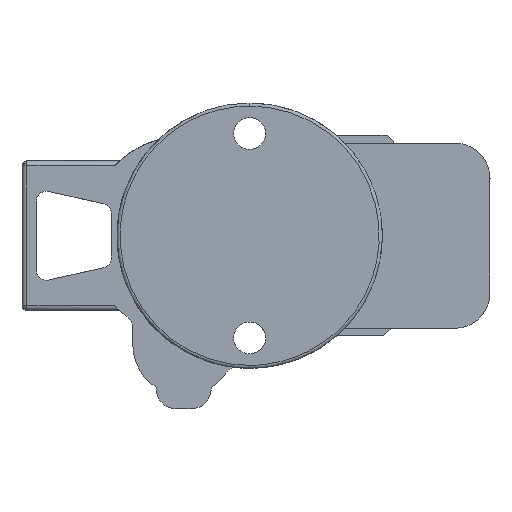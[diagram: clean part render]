
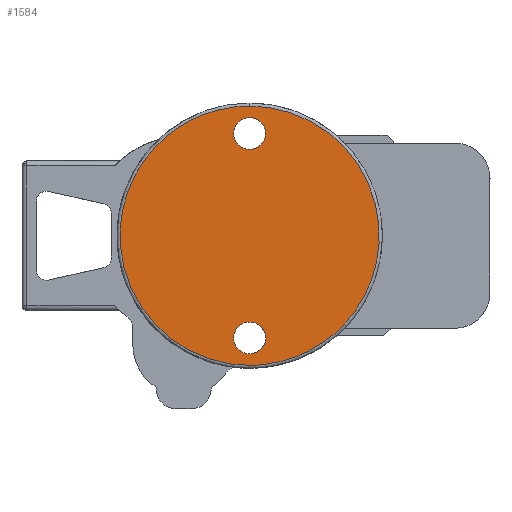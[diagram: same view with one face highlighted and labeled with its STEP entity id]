
A CAD part, left-side view. The second image highlights one B-rep face of the part: STEP entity #1584.
In plain terms, the highlighted planar face has unit normal (-1, 0, 0).
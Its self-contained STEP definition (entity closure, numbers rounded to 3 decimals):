
#74 = DIRECTION ( 'NONE',  ( 0., 0., -1. ) ) ;
#78 = VERTEX_POINT ( 'NONE', #683 ) ;
#122 = ORIENTED_EDGE ( 'NONE', *, *, #135, .F. ) ;
#135 = EDGE_CURVE ( 'NONE', #78, #2031, #2681, .T. ) ;
#228 = CARTESIAN_POINT ( 'NONE',  ( -218.682, 34.658, -22.7 ) ) ;
#279 = CARTESIAN_POINT ( 'NONE',  ( -218.682, 34.658, 18.3 ) ) ;
#391 = DIRECTION ( 'NONE',  ( -1., 0., 0. ) ) ;
#437 = CARTESIAN_POINT ( 'NONE',  ( -218.682, 34.658, -16.3 ) ) ;
#619 =( BOUNDED_CURVE ( )  B_SPLINE_CURVE ( 3, ( #1384, #3338, #1368, #3068 ),
 .UNSPECIFIED., .F., .T. ) 
 B_SPLINE_CURVE_WITH_KNOTS ( ( 4, 4 ),
 ( 0.876, 1.376 ),
 .UNSPECIFIED. ) 
 CURVE ( )  GEOMETRIC_REPRESENTATION_ITEM ( )  RATIONAL_B_SPLINE_CURVE ( ( 1., 0.333, 0.333, 1. ) ) 
 REPRESENTATION_ITEM ( '' )  );
#683 = CARTESIAN_POINT ( 'NONE',  ( -218.682, 34.658, 24.7 ) ) ;
#753 = AXIS2_PLACEMENT_3D ( 'NONE', #2430, #1034, #2156 ) ;
#888 = AXIS2_PLACEMENT_3D ( 'NONE', #3192, #2886, #1496 ) ;
#916 = DIRECTION ( 'NONE',  ( 0., 0., -1. ) ) ;
#926 = EDGE_CURVE ( 'NONE', #2140, #1071, #619, .T. ) ;
#1034 = DIRECTION ( 'NONE',  ( -1., 0., 0. ) ) ;
#1071 = VERTEX_POINT ( 'NONE', #3484 ) ;
#1086 = EDGE_LOOP ( 'NONE', ( #3415, #3290 ) ) ;
#1128 = CARTESIAN_POINT ( 'NONE',  ( -218.682, 34.658, 21.5 ) ) ;
#1136 = DIRECTION ( 'NONE',  ( 0., 0., -1. ) ) ;
#1143 = ORIENTED_EDGE ( 'NONE', *, *, #3253, .F. ) ;
#1180 = FACE_BOUND ( 'NONE', #1340, .T. ) ;
#1198 = PLANE ( 'NONE',  #3098 ) ;
#1291 = EDGE_CURVE ( 'NONE', #1765, #1603, #2693, .T. ) ;
#1315 =( BOUNDED_CURVE ( )  B_SPLINE_CURVE ( 3, ( #3286, #3069, #3339, #2214 ),
 .UNSPECIFIED., .F., .T. ) 
 B_SPLINE_CURVE_WITH_KNOTS ( ( 4, 4 ),
 ( 0.376, 0.876 ),
 .UNSPECIFIED. ) 
 CURVE ( )  GEOMETRIC_REPRESENTATION_ITEM ( )  RATIONAL_B_SPLINE_CURVE ( ( 1., 0.333, 0.333, 1. ) ) 
 REPRESENTATION_ITEM ( '' )  );
#1340 = EDGE_LOOP ( 'NONE', ( #122, #2192 ) ) ;
#1368 = CARTESIAN_POINT ( 'NONE',  ( -218.682, 86.64, 26.991 ) ) ;
#1384 = CARTESIAN_POINT ( 'NONE',  ( -218.682, 34.658, -24.991 ) ) ;
#1496 = DIRECTION ( 'NONE',  ( 0., 0., -1. ) ) ;
#1584 = ADVANCED_FACE ( 'NONE', ( #2590, #1180, #2296 ), #1198, .F. ) ;
#1603 = VERTEX_POINT ( 'NONE', #437 ) ;
#1614 = CARTESIAN_POINT ( 'NONE',  ( -218.682, 34.658, -24.991 ) ) ;
#1765 = VERTEX_POINT ( 'NONE', #228 ) ;
#1886 = CIRCLE ( 'NONE', #888, 3.2 ) ;
#2031 = VERTEX_POINT ( 'NONE', #279 ) ;
#2140 = VERTEX_POINT ( 'NONE', #1614 ) ;
#2156 = DIRECTION ( 'NONE',  ( 0., 0., -1. ) ) ;
#2160 = AXIS2_PLACEMENT_3D ( 'NONE', #3302, #3014, #1136 ) ;
#2182 = AXIS2_PLACEMENT_3D ( 'NONE', #1128, #391, #74 ) ;
#2192 = ORIENTED_EDGE ( 'NONE', *, *, #2774, .F. ) ;
#2214 = CARTESIAN_POINT ( 'NONE',  ( -218.682, 34.658, -24.991 ) ) ;
#2296 = FACE_BOUND ( 'NONE', #2443, .T. ) ;
#2311 = CARTESIAN_POINT ( 'NONE',  ( -218.682, 8.067, 1. ) ) ;
#2424 = ORIENTED_EDGE ( 'NONE', *, *, #1291, .F. ) ;
#2430 = CARTESIAN_POINT ( 'NONE',  ( -218.682, 34.658, -19.5 ) ) ;
#2443 = EDGE_LOOP ( 'NONE', ( #1143, #2424 ) ) ;
#2485 = EDGE_CURVE ( 'NONE', #1071, #2140, #1315, .T. ) ;
#2590 = FACE_OUTER_BOUND ( 'NONE', #1086, .T. ) ;
#2681 = CIRCLE ( 'NONE', #2160, 3.2 ) ;
#2693 = CIRCLE ( 'NONE', #753, 3.2 ) ;
#2774 = EDGE_CURVE ( 'NONE', #2031, #78, #3518, .T. ) ;
#2886 = DIRECTION ( 'NONE',  ( -1., 0., 0. ) ) ;
#3014 = DIRECTION ( 'NONE',  ( -1., 0., 0. ) ) ;
#3068 = CARTESIAN_POINT ( 'NONE',  ( -218.682, 34.658, 26.991 ) ) ;
#3069 = CARTESIAN_POINT ( 'NONE',  ( -218.682, -17.323, 26.991 ) ) ;
#3098 = AXIS2_PLACEMENT_3D ( 'NONE', #2311, #3422, #916 ) ;
#3192 = CARTESIAN_POINT ( 'NONE',  ( -218.682, 34.658, -19.5 ) ) ;
#3253 = EDGE_CURVE ( 'NONE', #1603, #1765, #1886, .T. ) ;
#3286 = CARTESIAN_POINT ( 'NONE',  ( -218.682, 34.658, 26.991 ) ) ;
#3290 = ORIENTED_EDGE ( 'NONE', *, *, #926, .F. ) ;
#3302 = CARTESIAN_POINT ( 'NONE',  ( -218.682, 34.658, 21.5 ) ) ;
#3338 = CARTESIAN_POINT ( 'NONE',  ( -218.682, 86.64, -24.991 ) ) ;
#3339 = CARTESIAN_POINT ( 'NONE',  ( -218.682, -17.323, -24.991 ) ) ;
#3415 = ORIENTED_EDGE ( 'NONE', *, *, #2485, .F. ) ;
#3422 = DIRECTION ( 'NONE',  ( 1., 0., 0. ) ) ;
#3484 = CARTESIAN_POINT ( 'NONE',  ( -218.682, 34.658, 26.991 ) ) ;
#3518 = CIRCLE ( 'NONE', #2182, 3.2 ) ;
